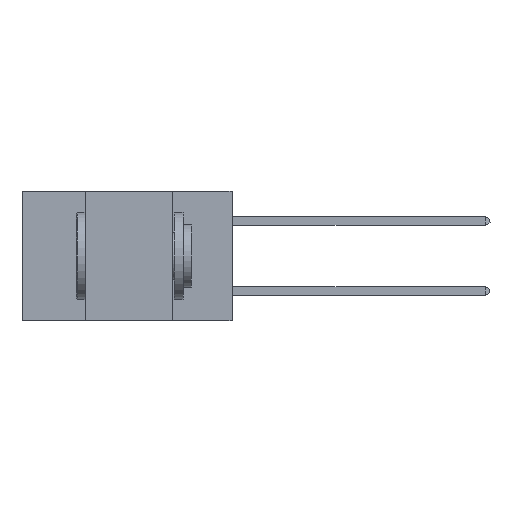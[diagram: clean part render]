
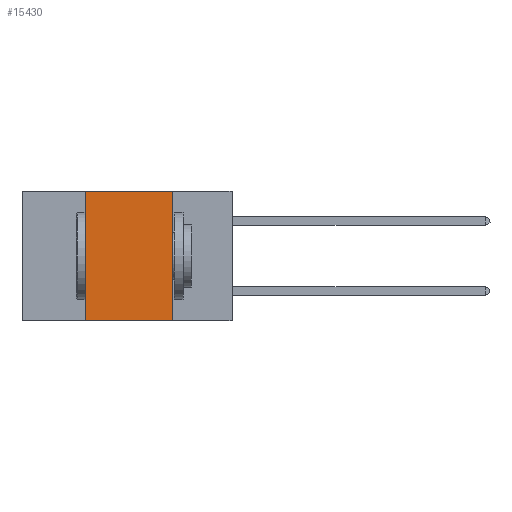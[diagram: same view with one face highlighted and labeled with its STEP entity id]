
A CAD part, left-side view. The second image highlights one B-rep face of the part: STEP entity #15430.
In plain terms, the highlighted planar face has unit normal (-1, 0, 0).
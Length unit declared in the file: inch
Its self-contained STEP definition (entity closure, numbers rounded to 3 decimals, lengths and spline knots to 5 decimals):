
#148 = CARTESIAN_POINT ( 'NONE',  ( 0., 0.6, 0. ) ) ;
#206 = LINE ( 'NONE', #14417, #15538 ) ;
#266 = CARTESIAN_POINT ( 'NONE',  ( 0., 0.42, 0. ) ) ;
#1167 = EDGE_CURVE ( 'NONE', #12295, #1466, #18280, .T. ) ;
#1466 = VERTEX_POINT ( 'NONE', #16000 ) ;
#1803 = DIRECTION ( 'NONE',  ( 1., 0., 0. ) ) ;
#3364 = DIRECTION ( 'NONE',  ( 0., 0., -1. ) ) ;
#4026 = LINE ( 'NONE', #7091, #10515 ) ;
#6141 = DIRECTION ( 'NONE',  ( 0., -1., 0. ) ) ;
#6354 = VECTOR ( 'NONE', #13505, 39.37008 ) ;
#6746 = EDGE_CURVE ( 'NONE', #1466, #13520, #12859, .T. ) ;
#7091 = CARTESIAN_POINT ( 'NONE',  ( 0., 0.6, -0.37 ) ) ;
#7407 = EDGE_CURVE ( 'NONE', #17723, #13520, #4026, .T. ) ;
#8066 = VECTOR ( 'NONE', #6141, 39.37008 ) ;
#8662 = CARTESIAN_POINT ( 'NONE',  ( 0., 0.17, -0.37 ) ) ;
#9039 = AXIS2_PLACEMENT_3D ( 'NONE', #10686, #1803, #3364 ) ;
#10006 = CARTESIAN_POINT ( 'NONE',  ( 0., 0.42, -0.37 ) ) ;
#10515 = VECTOR ( 'NONE', #18036, 39.37008 ) ;
#10686 = CARTESIAN_POINT ( 'NONE',  ( 0., 0.6, 0. ) ) ;
#11146 = ORIENTED_EDGE ( 'NONE', *, *, #1167, .F. ) ;
#11459 = EDGE_LOOP ( 'NONE', ( #19102, #11146, #12685, #13915 ) ) ;
#12295 = VERTEX_POINT ( 'NONE', #266 ) ;
#12685 = ORIENTED_EDGE ( 'NONE', *, *, #18903, .F. ) ;
#12859 = LINE ( 'NONE', #17927, #6354 ) ;
#13487 = PLANE ( 'NONE',  #9039 ) ;
#13505 = DIRECTION ( 'NONE',  ( 0., 0., -1. ) ) ;
#13520 = VERTEX_POINT ( 'NONE', #8662 ) ;
#13915 = ORIENTED_EDGE ( 'NONE', *, *, #7407, .T. ) ;
#14417 = CARTESIAN_POINT ( 'NONE',  ( 0., 0.42, 0. ) ) ;
#14438 = FACE_OUTER_BOUND ( 'NONE', #11459, .T. ) ;
#15430 = ADVANCED_FACE ( 'NONE', ( #14438 ), #13487, .F. ) ;
#15538 = VECTOR ( 'NONE', #18574, 39.37008 ) ;
#16000 = CARTESIAN_POINT ( 'NONE',  ( 0., 0.17, 0. ) ) ;
#17723 = VERTEX_POINT ( 'NONE', #10006 ) ;
#17927 = CARTESIAN_POINT ( 'NONE',  ( 0., 0.17, 0. ) ) ;
#18036 = DIRECTION ( 'NONE',  ( 0., -1., 0. ) ) ;
#18280 = LINE ( 'NONE', #148, #8066 ) ;
#18574 = DIRECTION ( 'NONE',  ( 0., 0., 1. ) ) ;
#18903 = EDGE_CURVE ( 'NONE', #17723, #12295, #206, .T. ) ;
#19102 = ORIENTED_EDGE ( 'NONE', *, *, #6746, .F. ) ;
